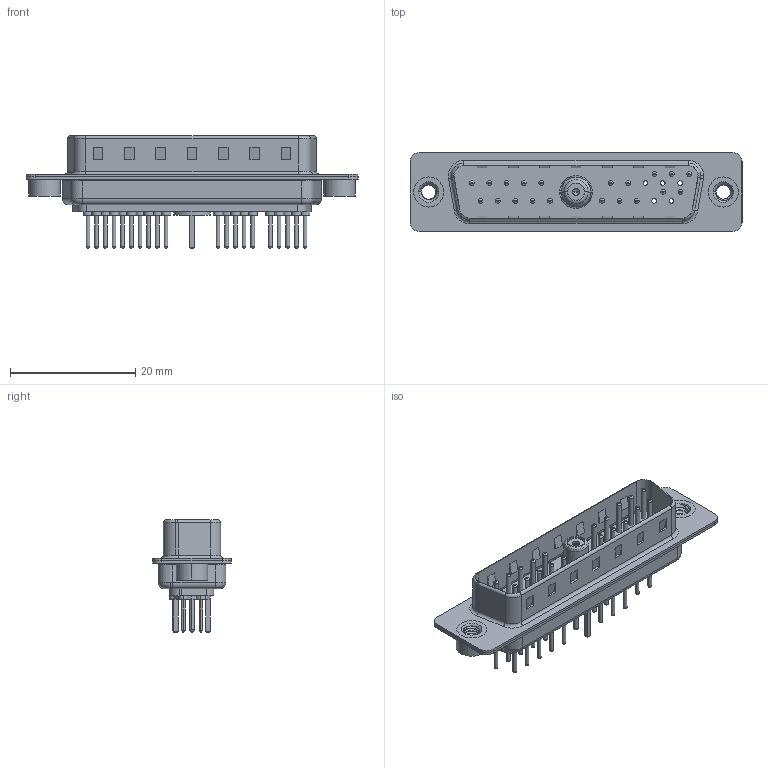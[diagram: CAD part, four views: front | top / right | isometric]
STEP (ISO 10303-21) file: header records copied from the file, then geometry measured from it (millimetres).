
FILE_DESCRIPTION (( 'STEP AP203' ), '1' );
FILE_NAME ('627-21W1224-7TA.STEP', '2019-05-28T01:01:42', ( '' ), ( '' ), 'SwSTEP 2.0', 'SolidWorks 2016', '' );
FILE_SCHEMA (( 'CONFIG_CONTROL_DESIGN' ));
Length unit declared in the file: millimetre
Products named in the file (14): 627Combo Threaded Rivet_A; Co-Ax Jack Assy_S; 627Combo Contact Row 1_24; Insulator Socket 2; 627Combo Housing_21W1; 627Combo Contact Row 2_24; Insulator Socket; 627Combo Shell Front_25 Contacts; 627-21W1224-7TA; Co-Ax Jack_Straight PC Tail; 627Combo Threaded Rivet_2; 627Combo Shell Rear_25 Contacts; Socket_Str; Locking Collar
Assembly tree (31 placements, depth 3):
  627-21W1224-7TA
    627Combo Housing_21W1
    627Combo Shell Rear_25 Contacts
    627Combo Shell Front_25 Contacts
    627Combo Threaded Rivet_A
    Co-Ax Jack Assy_S
      Co-Ax Jack_Straight PC Tail
      Insulator Socket
      Insulator Socket 2
      Locking Collar
      Socket_Str
    627Combo Threaded Rivet_2
    627Combo Contact Row 1_24  x10
    627Combo Contact Row 2_24  x10
Bounding box: 53 x 12.6 x 17.9 mm (x, y, z)
Volume: 2741.1 mm3; surface area: 7231 mm2
Topology: 30 solids, 30 shells, 1226 faces, 2683 edges, 1636 vertices
Faces by surface type: cylinder 465, torus 374, plane 358, cone 19, bspline 8, sphere 2
Entity records: 25840 total; most frequent: CARTESIAN_POINT 6897, DIRECTION 3811, ORIENTED_EDGE 3338, EDGE_CURVE 1669, AXIS2_PLACEMENT_3D 1502, VERTEX_POINT 1060, EDGE_LOOP 867, VECTOR 807
